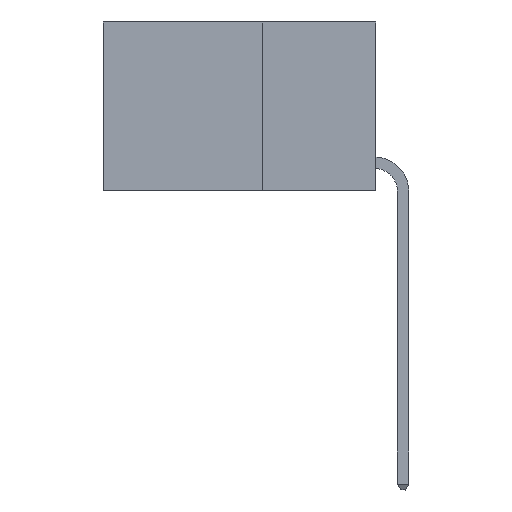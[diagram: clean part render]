
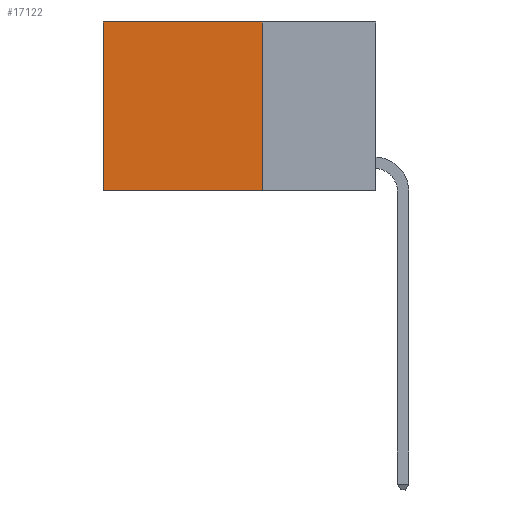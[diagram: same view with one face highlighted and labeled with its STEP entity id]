
A CAD part, left-side view. The second image highlights one B-rep face of the part: STEP entity #17122.
In plain terms, the highlighted planar face has unit normal (-1, 0, 0).
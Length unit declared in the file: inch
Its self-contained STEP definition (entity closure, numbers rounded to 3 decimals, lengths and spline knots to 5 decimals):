
#2698 = CARTESIAN_POINT ( 'NONE',  ( 0.2625, 0.25, 0. ) ) ;
#3653 = EDGE_CURVE ( 'NONE', #14426, #5075, #16541, .T. ) ;
#4279 = VECTOR ( 'NONE', #21366, 39.37008 ) ;
#4514 = DIRECTION ( 'NONE',  ( 0., 0., -1. ) ) ;
#5075 = VERTEX_POINT ( 'NONE', #7880 ) ;
#5275 = ORIENTED_EDGE ( 'NONE', *, *, #7137, .T. ) ;
#7066 = CARTESIAN_POINT ( 'NONE',  ( 0.2625, 0.25, 0. ) ) ;
#7137 = EDGE_CURVE ( 'NONE', #15388, #18891, #21438, .T. ) ;
#7748 = VECTOR ( 'NONE', #12613, 39.37008 ) ;
#7880 = CARTESIAN_POINT ( 'NONE',  ( 0.2625, 0.6, -0.37 ) ) ;
#8295 = FACE_OUTER_BOUND ( 'NONE', #10856, .T. ) ;
#10856 = EDGE_LOOP ( 'NONE', ( #11849, #17299, #22378, #5275 ) ) ;
#11212 = EDGE_CURVE ( 'NONE', #15388, #14426, #18570, .T. ) ;
#11849 = ORIENTED_EDGE ( 'NONE', *, *, #17604, .T. ) ;
#12613 = DIRECTION ( 'NONE',  ( 0., 1., 0. ) ) ;
#14426 = VERTEX_POINT ( 'NONE', #22821 ) ;
#14719 = CARTESIAN_POINT ( 'NONE',  ( 0.2625, 0.6, 0. ) ) ;
#14829 = DIRECTION ( 'NONE',  ( 0., 0., -1. ) ) ;
#15217 = DIRECTION ( 'NONE',  ( 1., 0., 0. ) ) ;
#15388 = VERTEX_POINT ( 'NONE', #19457 ) ;
#16541 = LINE ( 'NONE', #23012, #20722 ) ;
#16562 = CARTESIAN_POINT ( 'NONE',  ( 0.2625, 0.6, 0. ) ) ;
#17122 = ADVANCED_FACE ( 'NONE', ( #8295 ), #20556, .F. ) ;
#17299 = ORIENTED_EDGE ( 'NONE', *, *, #3653, .F. ) ;
#17604 = EDGE_CURVE ( 'NONE', #18891, #5075, #21968, .T. ) ;
#18570 = LINE ( 'NONE', #7066, #4279 ) ;
#18891 = VERTEX_POINT ( 'NONE', #14719 ) ;
#19457 = CARTESIAN_POINT ( 'NONE',  ( 0.2625, 0.25, 0. ) ) ;
#20444 = AXIS2_PLACEMENT_3D ( 'NONE', #2698, #15217, #4514 ) ;
#20556 = PLANE ( 'NONE',  #20444 ) ;
#20722 = VECTOR ( 'NONE', #22891, 39.37008 ) ;
#20851 = VECTOR ( 'NONE', #14829, 39.37008 ) ;
#21366 = DIRECTION ( 'NONE',  ( 0., 0., -1. ) ) ;
#21438 = LINE ( 'NONE', #21544, #7748 ) ;
#21544 = CARTESIAN_POINT ( 'NONE',  ( 0.2625, 0.25, 0. ) ) ;
#21968 = LINE ( 'NONE', #16562, #20851 ) ;
#22378 = ORIENTED_EDGE ( 'NONE', *, *, #11212, .F. ) ;
#22821 = CARTESIAN_POINT ( 'NONE',  ( 0.2625, 0.25, -0.37 ) ) ;
#22891 = DIRECTION ( 'NONE',  ( 0., 1., 0. ) ) ;
#23012 = CARTESIAN_POINT ( 'NONE',  ( 0.2625, 0.25, -0.37 ) ) ;
